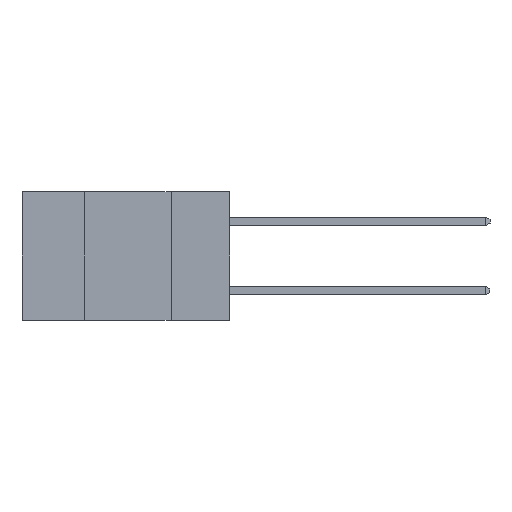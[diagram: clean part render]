
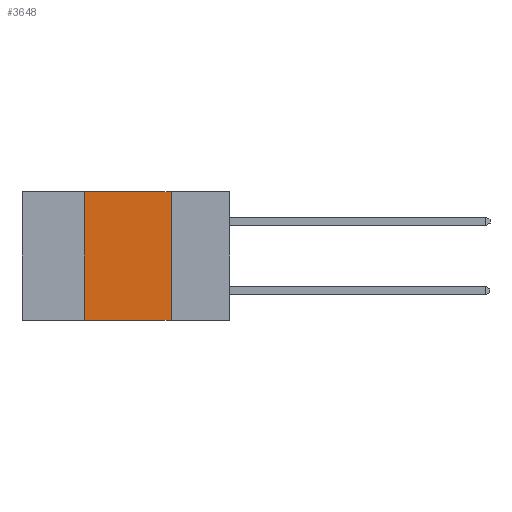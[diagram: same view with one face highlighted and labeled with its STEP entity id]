
A CAD part, left-side view. The second image highlights one B-rep face of the part: STEP entity #3648.
In plain terms, the highlighted planar face has unit normal (-1, 0, 0).
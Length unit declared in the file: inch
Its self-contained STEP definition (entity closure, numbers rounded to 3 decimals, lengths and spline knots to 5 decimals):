
#22 = VERTEX_POINT ( 'NONE', #4836 ) ;
#690 = CARTESIAN_POINT ( 'NONE',  ( 0., 0.6, -0.37 ) ) ;
#770 = DIRECTION ( 'NONE',  ( 0., 0., -1. ) ) ;
#1446 = CARTESIAN_POINT ( 'NONE',  ( 0., 0.42, -0.37 ) ) ;
#1582 = LINE ( 'NONE', #9104, #10004 ) ;
#1613 = DIRECTION ( 'NONE',  ( 0., -1., 0. ) ) ;
#2556 = CARTESIAN_POINT ( 'NONE',  ( 0., 0.42, 0. ) ) ;
#2750 = VERTEX_POINT ( 'NONE', #1446 ) ;
#2753 = VECTOR ( 'NONE', #9932, 39.37008 ) ;
#2906 = CARTESIAN_POINT ( 'NONE',  ( 0., 0.42, 0. ) ) ;
#3054 = LINE ( 'NONE', #7673, #2753 ) ;
#3648 = ADVANCED_FACE ( 'NONE', ( #7309 ), #8730, .F. ) ;
#4087 = ORIENTED_EDGE ( 'NONE', *, *, #6024, .T. ) ;
#4388 = EDGE_CURVE ( 'NONE', #7927, #22, #3054, .T. ) ;
#4402 = DIRECTION ( 'NONE',  ( 0., 0., -1. ) ) ;
#4625 = VECTOR ( 'NONE', #6765, 39.37008 ) ;
#4836 = CARTESIAN_POINT ( 'NONE',  ( 0., 0.17, 0. ) ) ;
#4920 = EDGE_CURVE ( 'NONE', #22, #6053, #1582, .T. ) ;
#5483 = EDGE_CURVE ( 'NONE', #2750, #7927, #7026, .T. ) ;
#5503 = AXIS2_PLACEMENT_3D ( 'NONE', #7535, #9129, #4402 ) ;
#6024 = EDGE_CURVE ( 'NONE', #2750, #6053, #10353, .T. ) ;
#6053 = VERTEX_POINT ( 'NONE', #6788 ) ;
#6765 = DIRECTION ( 'NONE',  ( 0., 0., 1. ) ) ;
#6788 = CARTESIAN_POINT ( 'NONE',  ( 0., 0.17, -0.37 ) ) ;
#7026 = LINE ( 'NONE', #2556, #4625 ) ;
#7309 = FACE_OUTER_BOUND ( 'NONE', #8315, .T. ) ;
#7478 = ORIENTED_EDGE ( 'NONE', *, *, #4920, .F. ) ;
#7535 = CARTESIAN_POINT ( 'NONE',  ( 0., 0.6, 0. ) ) ;
#7673 = CARTESIAN_POINT ( 'NONE',  ( 0., 0.6, 0. ) ) ;
#7845 = ORIENTED_EDGE ( 'NONE', *, *, #4388, .F. ) ;
#7927 = VERTEX_POINT ( 'NONE', #2906 ) ;
#8315 = EDGE_LOOP ( 'NONE', ( #7478, #7845, #10076, #4087 ) ) ;
#8730 = PLANE ( 'NONE',  #5503 ) ;
#9104 = CARTESIAN_POINT ( 'NONE',  ( 0., 0.17, 0. ) ) ;
#9129 = DIRECTION ( 'NONE',  ( 1., 0., 0. ) ) ;
#9910 = VECTOR ( 'NONE', #1613, 39.37008 ) ;
#9932 = DIRECTION ( 'NONE',  ( 0., -1., 0. ) ) ;
#10004 = VECTOR ( 'NONE', #770, 39.37008 ) ;
#10076 = ORIENTED_EDGE ( 'NONE', *, *, #5483, .F. ) ;
#10353 = LINE ( 'NONE', #690, #9910 ) ;
